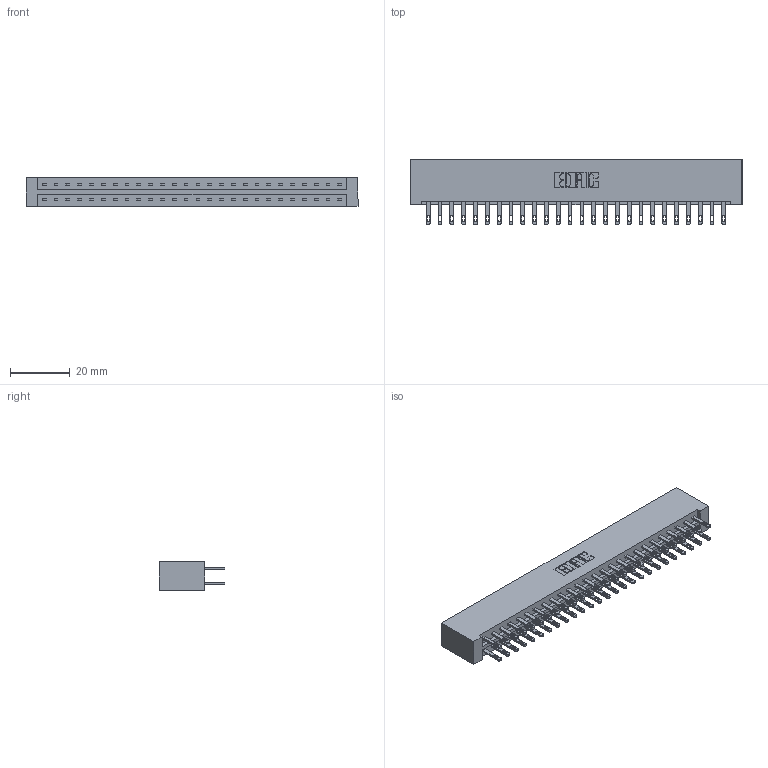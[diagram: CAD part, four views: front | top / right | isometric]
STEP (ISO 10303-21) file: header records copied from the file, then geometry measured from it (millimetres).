
FILE_DESCRIPTION (( 'STEP AP203' ), '1' );
FILE_NAME ('333-052-500-201.STEP', '2018-08-04T01:42:29', ( '' ), ( '' ), 'SwSTEP 2.0', 'SolidWorks 2016', '' );
FILE_SCHEMA (( 'CONFIG_CONTROL_DESIGN' ));
Length unit declared in the file: inch
Products named in the file (3): 333 Part_Lugless; 345-292-001_345-293-100; 333-052-500-201
Assembly tree (53 placements, depth 2):
  333-052-500-201
    333 Part_Lugless
    345-292-001_345-293-100  x52
Bounding box: 111.28 x 21.85 x 9.4 mm (x, y, z)
Volume: 12002.3 mm3; surface area: 14614.3 mm2
Topology: 53 solids, 53 shells, 2602 faces, 7931 edges, 5286 vertices
Faces by surface type: plane 1626, cylinder 976
Entity records: 18449 total; most frequent: CARTESIAN_POINT 3074, ORIENTED_EDGE 3010, DIRECTION 2649, EDGE_CURVE 1505, VECTOR 1381, LINE 1381, VERTEX_POINT 1002, AXIS2_PLACEMENT_3D 634
